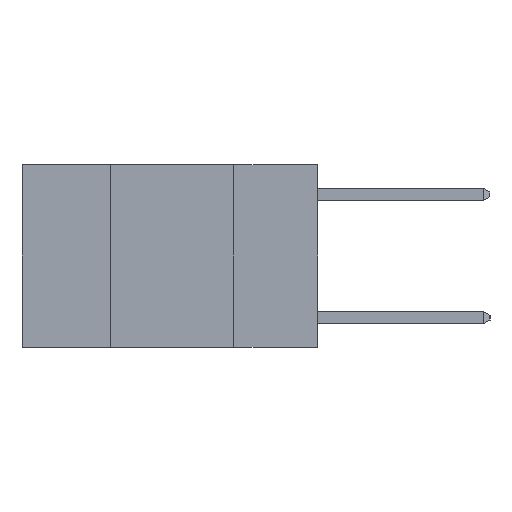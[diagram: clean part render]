
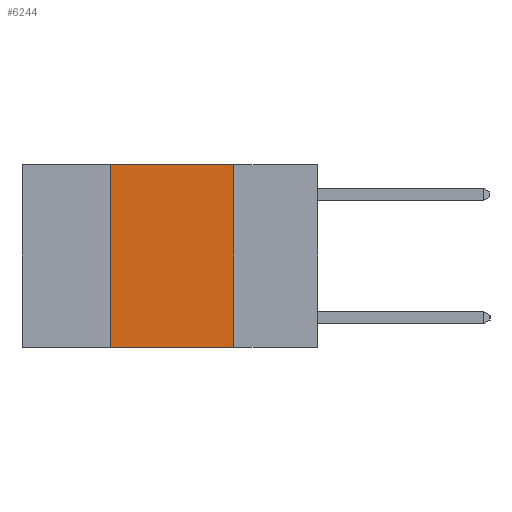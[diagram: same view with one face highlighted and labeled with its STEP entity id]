
A CAD part, left-side view. The second image highlights one B-rep face of the part: STEP entity #6244.
In plain terms, the highlighted planar face has unit normal (-1, 0, 0).
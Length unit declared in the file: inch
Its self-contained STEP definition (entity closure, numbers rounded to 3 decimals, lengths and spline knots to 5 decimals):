
#173 = VECTOR ( 'NONE', #9432, 39.37008 ) ;
#643 = EDGE_LOOP ( 'NONE', ( #6726, #2072, #7359, #5867 ) ) ;
#868 = LINE ( 'NONE', #8126, #9642 ) ;
#1566 = AXIS2_PLACEMENT_3D ( 'NONE', #7008, #2097, #7827 ) ;
#2053 = CARTESIAN_POINT ( 'NONE',  ( 0., 0.17, 0. ) ) ;
#2072 = ORIENTED_EDGE ( 'NONE', *, *, #9606, .F. ) ;
#2097 = DIRECTION ( 'NONE',  ( 1., 0., 0. ) ) ;
#2427 = EDGE_CURVE ( 'NONE', #9717, #4659, #10631, .T. ) ;
#2895 = DIRECTION ( 'NONE',  ( 0., 0., -1. ) ) ;
#2977 = EDGE_CURVE ( 'NONE', #4727, #4659, #9236, .T. ) ;
#3204 = DIRECTION ( 'NONE',  ( 0., 0., 1. ) ) ;
#3641 = CARTESIAN_POINT ( 'NONE',  ( 0., 0.6, -0.37 ) ) ;
#3688 = CARTESIAN_POINT ( 'NONE',  ( 0., 0.6, 0. ) ) ;
#4505 = EDGE_CURVE ( 'NONE', #9717, #7281, #868, .T. ) ;
#4659 = VERTEX_POINT ( 'NONE', #5155 ) ;
#4727 = VERTEX_POINT ( 'NONE', #10210 ) ;
#5155 = CARTESIAN_POINT ( 'NONE',  ( 0., 0.17, -0.37 ) ) ;
#5326 = PLANE ( 'NONE',  #1566 ) ;
#5657 = LINE ( 'NONE', #3688, #7878 ) ;
#5867 = ORIENTED_EDGE ( 'NONE', *, *, #2427, .T. ) ;
#6244 = ADVANCED_FACE ( 'NONE', ( #7499 ), #5326, .F. ) ;
#6726 = ORIENTED_EDGE ( 'NONE', *, *, #2977, .F. ) ;
#7008 = CARTESIAN_POINT ( 'NONE',  ( 0., 0.6, 0. ) ) ;
#7258 = VECTOR ( 'NONE', #2895, 39.37008 ) ;
#7281 = VERTEX_POINT ( 'NONE', #8216 ) ;
#7359 = ORIENTED_EDGE ( 'NONE', *, *, #4505, .F. ) ;
#7499 = FACE_OUTER_BOUND ( 'NONE', #643, .T. ) ;
#7809 = DIRECTION ( 'NONE',  ( 0., -1., 0. ) ) ;
#7827 = DIRECTION ( 'NONE',  ( 0., 0., -1. ) ) ;
#7878 = VECTOR ( 'NONE', #7809, 39.37008 ) ;
#8126 = CARTESIAN_POINT ( 'NONE',  ( 0., 0.42, 0. ) ) ;
#8216 = CARTESIAN_POINT ( 'NONE',  ( 0., 0.42, 0. ) ) ;
#9236 = LINE ( 'NONE', #2053, #7258 ) ;
#9432 = DIRECTION ( 'NONE',  ( 0., -1., 0. ) ) ;
#9606 = EDGE_CURVE ( 'NONE', #7281, #4727, #5657, .T. ) ;
#9642 = VECTOR ( 'NONE', #3204, 39.37008 ) ;
#9717 = VERTEX_POINT ( 'NONE', #10412 ) ;
#10210 = CARTESIAN_POINT ( 'NONE',  ( 0., 0.17, 0. ) ) ;
#10412 = CARTESIAN_POINT ( 'NONE',  ( 0., 0.42, -0.37 ) ) ;
#10631 = LINE ( 'NONE', #3641, #173 ) ;
